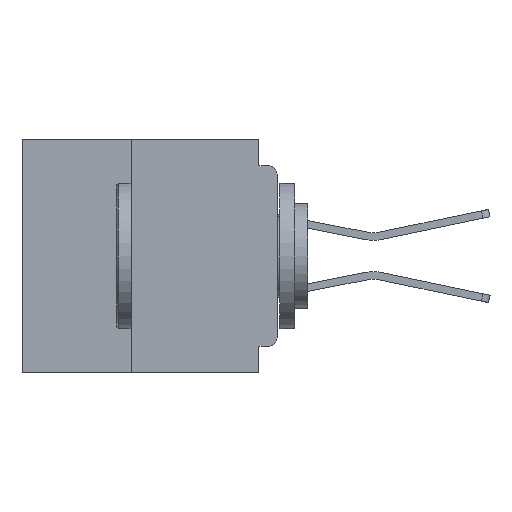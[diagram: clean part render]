
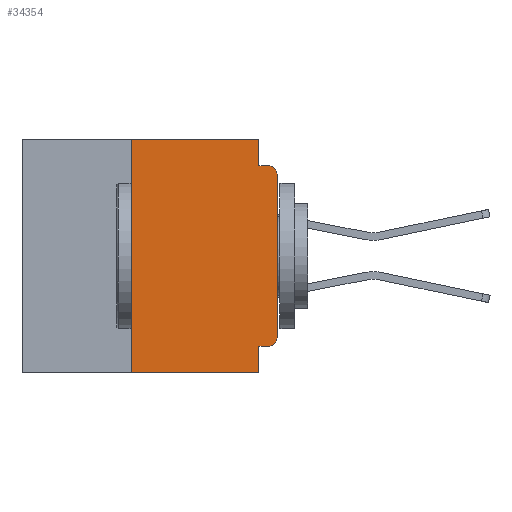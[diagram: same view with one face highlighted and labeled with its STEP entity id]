
A CAD part, left-side view. The second image highlights one B-rep face of the part: STEP entity #34354.
In plain terms, the highlighted planar face has unit normal (-1, 0, 0).
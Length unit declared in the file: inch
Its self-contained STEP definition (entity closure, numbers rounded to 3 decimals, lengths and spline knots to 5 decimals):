
#966 = DIRECTION ( 'NONE',  ( 0., -1., 0. ) ) ;
#1189 = EDGE_CURVE ( 'NONE', #51161, #11038, #56079, .T. ) ;
#1493 = CIRCLE ( 'NONE', #31584, 0.015 ) ;
#2076 = LINE ( 'NONE', #12274, #25710 ) ;
#2208 = ORIENTED_EDGE ( 'NONE', *, *, #21372, .F. ) ;
#4992 = CARTESIAN_POINT ( 'NONE',  ( 0., 0., -0.355 ) ) ;
#5065 = DIRECTION ( 'NONE',  ( 0., 0., 1. ) ) ;
#5259 = CARTESIAN_POINT ( 'NONE',  ( 0., 0.015, -0.34 ) ) ;
#5906 = CARTESIAN_POINT ( 'NONE',  ( 0., 0.031, 0. ) ) ;
#6232 = VERTEX_POINT ( 'NONE', #35802 ) ;
#6783 = CARTESIAN_POINT ( 'NONE',  ( 0., 0.015, -0.06 ) ) ;
#7601 = CIRCLE ( 'NONE', #30552, 0.015 ) ;
#7781 = LINE ( 'NONE', #46233, #31456 ) ;
#7956 = ORIENTED_EDGE ( 'NONE', *, *, #37121, .F. ) ;
#9140 = ORIENTED_EDGE ( 'NONE', *, *, #27091, .F. ) ;
#9995 = DIRECTION ( 'NONE',  ( 0., 0., -1. ) ) ;
#11038 = VERTEX_POINT ( 'NONE', #45898 ) ;
#11448 = FACE_OUTER_BOUND ( 'NONE', #11677, .T. ) ;
#11510 = DIRECTION ( 'NONE',  ( 0., 0., -1. ) ) ;
#11677 = EDGE_LOOP ( 'NONE', ( #15257, #39663, #2208, #9140, #45970, #55248, #25310, #20719, #7956, #31524 ) ) ;
#12274 = CARTESIAN_POINT ( 'NONE',  ( 0., 0.25, -0.4 ) ) ;
#12372 = VERTEX_POINT ( 'NONE', #32320 ) ;
#13857 = CARTESIAN_POINT ( 'NONE',  ( 0., 0.25, -0.4 ) ) ;
#14338 = CARTESIAN_POINT ( 'NONE',  ( 0., 0., 0. ) ) ;
#14954 = LINE ( 'NONE', #57066, #50865 ) ;
#15116 = LINE ( 'NONE', #14338, #26245 ) ;
#15257 = ORIENTED_EDGE ( 'NONE', *, *, #53538, .T. ) ;
#16911 = EDGE_CURVE ( 'NONE', #40060, #24508, #1493, .T. ) ;
#17617 = DIRECTION ( 'NONE',  ( 1., 0., 0. ) ) ;
#18994 = CARTESIAN_POINT ( 'NONE',  ( 0., 0., -0.06 ) ) ;
#19398 = CARTESIAN_POINT ( 'NONE',  ( 0., 0.031, 0. ) ) ;
#19983 = VERTEX_POINT ( 'NONE', #19398 ) ;
#20719 = ORIENTED_EDGE ( 'NONE', *, *, #1189, .F. ) ;
#21372 = EDGE_CURVE ( 'NONE', #12372, #24508, #44012, .T. ) ;
#24508 = VERTEX_POINT ( 'NONE', #38925 ) ;
#25310 = ORIENTED_EDGE ( 'NONE', *, *, #55838, .T. ) ;
#25710 = VECTOR ( 'NONE', #54426, 39.37008 ) ;
#25868 = LINE ( 'NONE', #5906, #50654 ) ;
#26245 = VECTOR ( 'NONE', #5065, 39.37008 ) ;
#26750 = CARTESIAN_POINT ( 'NONE',  ( 0., 0., -0.34 ) ) ;
#26946 = CARTESIAN_POINT ( 'NONE',  ( 0., 0.437, 0. ) ) ;
#27091 = EDGE_CURVE ( 'NONE', #19983, #12372, #25868, .T. ) ;
#30200 = VECTOR ( 'NONE', #40375, 39.37008 ) ;
#30546 = VECTOR ( 'NONE', #56355, 39.37008 ) ;
#30552 = AXIS2_PLACEMENT_3D ( 'NONE', #5259, #38168, #9995 ) ;
#31456 = VECTOR ( 'NONE', #50882, 39.37008 ) ;
#31524 = ORIENTED_EDGE ( 'NONE', *, *, #45576, .T. ) ;
#31584 = AXIS2_PLACEMENT_3D ( 'NONE', #6783, #39697, #11510 ) ;
#32320 = CARTESIAN_POINT ( 'NONE',  ( 0., 0.031, -0.045 ) ) ;
#34354 = ADVANCED_FACE ( 'NONE', ( #11448 ), #45699, .F. ) ;
#35802 = CARTESIAN_POINT ( 'NONE',  ( 0., 0.015, -0.355 ) ) ;
#35856 = EDGE_CURVE ( 'NONE', #38224, #19983, #14954, .T. ) ;
#36549 = CARTESIAN_POINT ( 'NONE',  ( 0., 0.031, -0.355 ) ) ;
#37121 = EDGE_CURVE ( 'NONE', #6232, #51161, #55235, .T. ) ;
#38168 = DIRECTION ( 'NONE',  ( -1., 0., 0. ) ) ;
#38224 = VERTEX_POINT ( 'NONE', #60504 ) ;
#38811 = DIRECTION ( 'NONE',  ( 0., 0., -1. ) ) ;
#38925 = CARTESIAN_POINT ( 'NONE',  ( 0., 0.015, -0.045 ) ) ;
#39049 = DIRECTION ( 'NONE',  ( 0., 0., -1. ) ) ;
#39469 = CARTESIAN_POINT ( 'NONE',  ( 0., 0.031, -0.4 ) ) ;
#39663 = ORIENTED_EDGE ( 'NONE', *, *, #16911, .T. ) ;
#39697 = DIRECTION ( 'NONE',  ( -1., 0., 0. ) ) ;
#40060 = VERTEX_POINT ( 'NONE', #18994 ) ;
#40375 = DIRECTION ( 'NONE',  ( 0., -1., 0. ) ) ;
#40926 = EDGE_CURVE ( 'NONE', #54140, #38224, #2076, .T. ) ;
#43761 = VECTOR ( 'NONE', #39049, 39.37008 ) ;
#44012 = LINE ( 'NONE', #49513, #30200 ) ;
#45576 = EDGE_CURVE ( 'NONE', #6232, #51085, #7601, .T. ) ;
#45699 = PLANE ( 'NONE',  #46548 ) ;
#45898 = CARTESIAN_POINT ( 'NONE',  ( 0., 0.031, -0.4 ) ) ;
#45970 = ORIENTED_EDGE ( 'NONE', *, *, #35856, .F. ) ;
#46233 = CARTESIAN_POINT ( 'NONE',  ( 0., 0.437, -0.4 ) ) ;
#46548 = AXIS2_PLACEMENT_3D ( 'NONE', #26946, #17617, #50359 ) ;
#49513 = CARTESIAN_POINT ( 'NONE',  ( 0., 0., -0.045 ) ) ;
#50359 = DIRECTION ( 'NONE',  ( 0., 0., -1. ) ) ;
#50654 = VECTOR ( 'NONE', #38811, 39.37008 ) ;
#50865 = VECTOR ( 'NONE', #966, 39.37008 ) ;
#50882 = DIRECTION ( 'NONE',  ( 0., -1., 0. ) ) ;
#51085 = VERTEX_POINT ( 'NONE', #26750 ) ;
#51161 = VERTEX_POINT ( 'NONE', #36549 ) ;
#53538 = EDGE_CURVE ( 'NONE', #51085, #40060, #15116, .T. ) ;
#54140 = VERTEX_POINT ( 'NONE', #13857 ) ;
#54426 = DIRECTION ( 'NONE',  ( 0., 0., 1. ) ) ;
#55235 = LINE ( 'NONE', #4992, #30546 ) ;
#55248 = ORIENTED_EDGE ( 'NONE', *, *, #40926, .F. ) ;
#55838 = EDGE_CURVE ( 'NONE', #54140, #11038, #7781, .T. ) ;
#56079 = LINE ( 'NONE', #39469, #43761 ) ;
#56355 = DIRECTION ( 'NONE',  ( 0., 1., 0. ) ) ;
#57066 = CARTESIAN_POINT ( 'NONE',  ( 0., 0.437, 0. ) ) ;
#60504 = CARTESIAN_POINT ( 'NONE',  ( 0., 0.25, 0. ) ) ;
